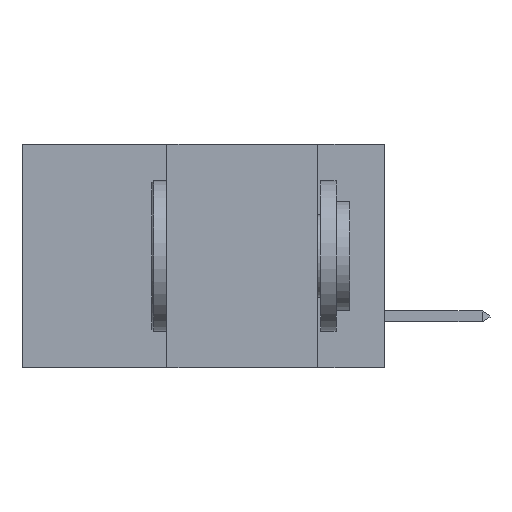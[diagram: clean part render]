
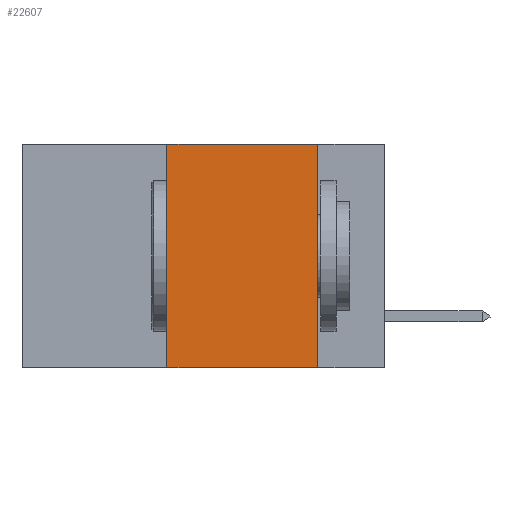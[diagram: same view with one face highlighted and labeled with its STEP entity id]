
A CAD part, left-side view. The second image highlights one B-rep face of the part: STEP entity #22607.
In plain terms, the highlighted planar face has unit normal (-1, 0, 0).
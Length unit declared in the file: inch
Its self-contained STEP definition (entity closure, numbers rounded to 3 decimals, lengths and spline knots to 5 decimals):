
#869 = ORIENTED_EDGE ( 'NONE', *, *, #11485, .T. ) ;
#1286 = ORIENTED_EDGE ( 'NONE', *, *, #22911, .F. ) ;
#2258 = CARTESIAN_POINT ( 'NONE',  ( 0., 0.11, -0.37 ) ) ;
#2336 = VERTEX_POINT ( 'NONE', #2258 ) ;
#2965 = AXIS2_PLACEMENT_3D ( 'NONE', #6642, #8838, #23564 ) ;
#3391 = DIRECTION ( 'NONE',  ( 0., -1., 0. ) ) ;
#3782 = VERTEX_POINT ( 'NONE', #4266 ) ;
#4266 = CARTESIAN_POINT ( 'NONE',  ( 0., 0.36, 0. ) ) ;
#4276 = CARTESIAN_POINT ( 'NONE',  ( 0., 0.6, -0.37 ) ) ;
#4369 = DIRECTION ( 'NONE',  ( 0., -1., 0. ) ) ;
#5519 = CARTESIAN_POINT ( 'NONE',  ( 0., 0.36, -0.37 ) ) ;
#6642 = CARTESIAN_POINT ( 'NONE',  ( 0., 0.6, 0. ) ) ;
#7115 = VECTOR ( 'NONE', #17241, 39.37008 ) ;
#7662 = VECTOR ( 'NONE', #9685, 39.37008 ) ;
#8358 = LINE ( 'NONE', #26502, #7662 ) ;
#8838 = DIRECTION ( 'NONE',  ( 1., 0., 0. ) ) ;
#9685 = DIRECTION ( 'NONE',  ( 0., 0., -1. ) ) ;
#11485 = EDGE_CURVE ( 'NONE', #20078, #2336, #27199, .T. ) ;
#12346 = VERTEX_POINT ( 'NONE', #15671 ) ;
#12903 = VECTOR ( 'NONE', #3391, 39.37008 ) ;
#14025 = ORIENTED_EDGE ( 'NONE', *, *, #23825, .F. ) ;
#14504 = EDGE_LOOP ( 'NONE', ( #26376, #1286, #14025, #869 ) ) ;
#15671 = CARTESIAN_POINT ( 'NONE',  ( 0., 0.11, 0. ) ) ;
#15897 = FACE_OUTER_BOUND ( 'NONE', #14504, .T. ) ;
#17241 = DIRECTION ( 'NONE',  ( 0., 0., 1. ) ) ;
#18503 = LINE ( 'NONE', #20382, #12903 ) ;
#19412 = PLANE ( 'NONE',  #2965 ) ;
#20025 = EDGE_CURVE ( 'NONE', #12346, #2336, #8358, .T. ) ;
#20078 = VERTEX_POINT ( 'NONE', #5519 ) ;
#20382 = CARTESIAN_POINT ( 'NONE',  ( 0., 0.6, 0. ) ) ;
#22607 = ADVANCED_FACE ( 'NONE', ( #15897 ), #19412, .F. ) ;
#22911 = EDGE_CURVE ( 'NONE', #3782, #12346, #18503, .T. ) ;
#23502 = CARTESIAN_POINT ( 'NONE',  ( 0., 0.36, 0. ) ) ;
#23564 = DIRECTION ( 'NONE',  ( 0., 0., -1. ) ) ;
#23825 = EDGE_CURVE ( 'NONE', #20078, #3782, #23977, .T. ) ;
#23977 = LINE ( 'NONE', #23502, #7115 ) ;
#26376 = ORIENTED_EDGE ( 'NONE', *, *, #20025, .F. ) ;
#26502 = CARTESIAN_POINT ( 'NONE',  ( 0., 0.11, 0. ) ) ;
#26543 = VECTOR ( 'NONE', #4369, 39.37008 ) ;
#27199 = LINE ( 'NONE', #4276, #26543 ) ;
